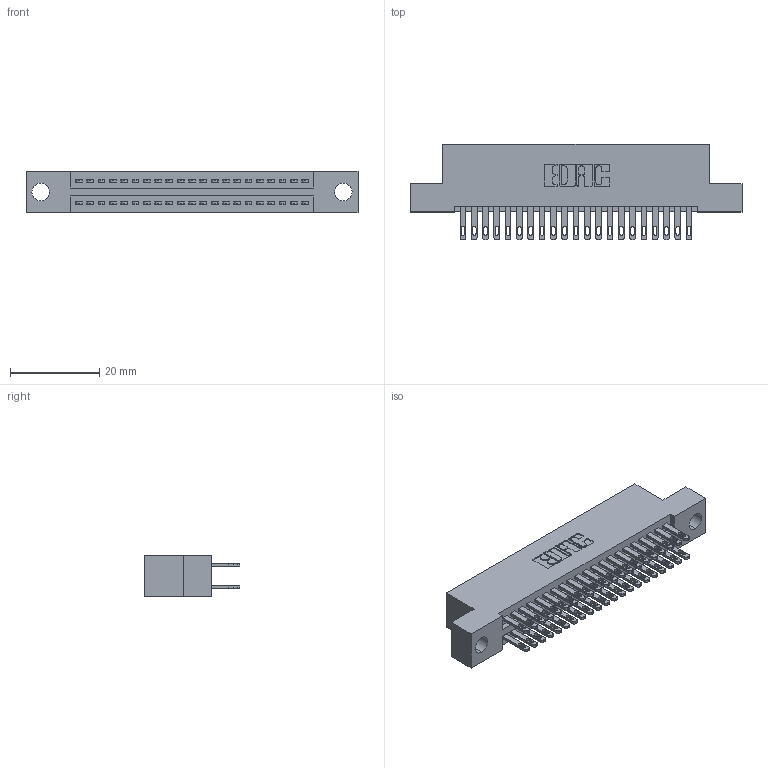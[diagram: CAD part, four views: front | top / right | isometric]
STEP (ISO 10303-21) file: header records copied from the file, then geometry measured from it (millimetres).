
FILE_DESCRIPTION (( 'STEP AP203' ), '1' );
FILE_NAME ('345-042-500-204.STEP', '2021-05-20T01:23:41', ( '' ), ( '' ), 'SwSTEP 2.0', 'SolidWorks 2020', '' );
FILE_SCHEMA (( 'CONFIG_CONTROL_DESIGN' ));
Length unit declared in the file: inch
Products named in the file (3): 345 Part_Flush Mounting Lugs - 0.156 Dia-TI; 345-292-001_345-293-100; 345-042-500-204
Assembly tree (43 placements, depth 2):
  345-042-500-204
    345 Part_Flush Mounting Lugs - 0.156 Dia-TI
    345-292-001_345-293-100  x42
Bounding box: 74.55 x 21.51 x 9.4 mm (x, y, z)
Volume: 7069.2 mm3; surface area: 10322.8 mm2
Topology: 43 solids, 43 shells, 2072 faces, 6299 edges, 4198 vertices
Faces by surface type: plane 1228, cylinder 844
Entity records: 19653 total; most frequent: CARTESIAN_POINT 3318, ORIENTED_EDGE 3250, DIRECTION 2953, EDGE_CURVE 1625, LINE 1405, VECTOR 1405, VERTEX_POINT 1082, AXIS2_PLACEMENT_3D 774
